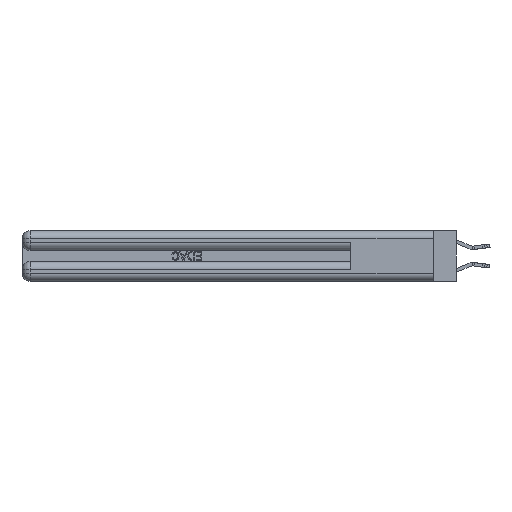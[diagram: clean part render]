
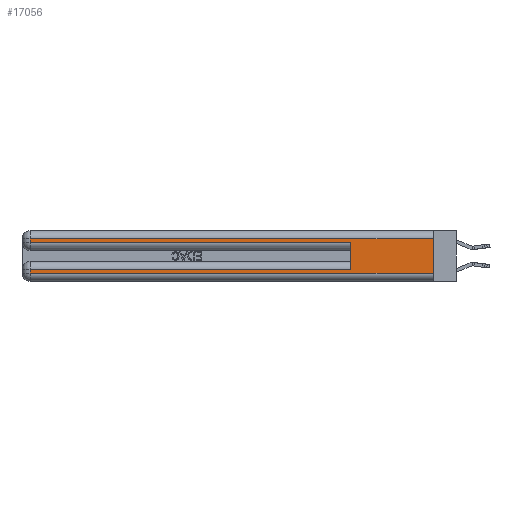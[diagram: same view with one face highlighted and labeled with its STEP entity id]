
A CAD part, left-side view. The second image highlights one B-rep face of the part: STEP entity #17056.
In plain terms, the highlighted planar face has unit normal (-1, 0, 0).
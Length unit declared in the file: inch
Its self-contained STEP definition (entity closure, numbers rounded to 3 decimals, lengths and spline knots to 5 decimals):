
#570 = CARTESIAN_POINT ( 'NONE',  ( 0., 0., 0.31 ) ) ;
#809 = DIRECTION ( 'NONE',  ( 0., -1., 0. ) ) ;
#1093 = LINE ( 'NONE', #29377, #14664 ) ;
#2727 = LINE ( 'NONE', #21797, #16278 ) ;
#3229 = CARTESIAN_POINT ( 'NONE',  ( 0., 0., 0.06 ) ) ;
#5122 = VECTOR ( 'NONE', #32197, 39.37008 ) ;
#5146 = ORIENTED_EDGE ( 'NONE', *, *, #20983, .T. ) ;
#5341 = CARTESIAN_POINT ( 'NONE',  ( 0., 0., 0.37 ) ) ;
#5838 = EDGE_CURVE ( 'NONE', #23781, #7945, #17142, .T. ) ;
#6413 = LINE ( 'NONE', #32430, #27212 ) ;
#6625 = LINE ( 'NONE', #570, #13001 ) ;
#7056 = CARTESIAN_POINT ( 'NONE',  ( 0., 2.94, 0.285 ) ) ;
#7945 = VERTEX_POINT ( 'NONE', #20571 ) ;
#8045 = DIRECTION ( 'NONE',  ( 0., 0., -1. ) ) ;
#8133 = VERTEX_POINT ( 'NONE', #23997 ) ;
#8464 = CARTESIAN_POINT ( 'NONE',  ( 0., 0., 0.285 ) ) ;
#8973 = FACE_OUTER_BOUND ( 'NONE', #31377, .T. ) ;
#9471 = ORIENTED_EDGE ( 'NONE', *, *, #14896, .T. ) ;
#10245 = VERTEX_POINT ( 'NONE', #3229 ) ;
#11460 = CARTESIAN_POINT ( 'NONE',  ( 0., 2.94, 0.085 ) ) ;
#13001 = VECTOR ( 'NONE', #16779, 39.37008 ) ;
#13388 = EDGE_CURVE ( 'NONE', #20049, #7945, #17546, .T. ) ;
#13820 = DIRECTION ( 'NONE',  ( 0., -1., 0. ) ) ;
#14614 = ORIENTED_EDGE ( 'NONE', *, *, #5838, .T. ) ;
#14664 = VECTOR ( 'NONE', #15831, 39.37008 ) ;
#14896 = EDGE_CURVE ( 'NONE', #8133, #23781, #6413, .T. ) ;
#15412 = CARTESIAN_POINT ( 'NONE',  ( 0., 0.6, 0.145 ) ) ;
#15568 = LINE ( 'NONE', #17002, #29161 ) ;
#15618 = EDGE_CURVE ( 'NONE', #28615, #20566, #2727, .T. ) ;
#15831 = DIRECTION ( 'NONE',  ( 0., 0., -1. ) ) ;
#16278 = VECTOR ( 'NONE', #24514, 39.37008 ) ;
#16779 = DIRECTION ( 'NONE',  ( 0., 1., 0. ) ) ;
#17002 = CARTESIAN_POINT ( 'NONE',  ( 0., 0., 0.06 ) ) ;
#17056 = ADVANCED_FACE ( 'NONE', ( #8973 ), #21589, .F. ) ;
#17142 = LINE ( 'NONE', #8464, #24382 ) ;
#17546 = LINE ( 'NONE', #15412, #23959 ) ;
#17814 = LINE ( 'NONE', #29443, #5122 ) ;
#18250 = CARTESIAN_POINT ( 'NONE',  ( 0., 0.6, 0.085 ) ) ;
#18718 = EDGE_CURVE ( 'NONE', #20049, #28615, #17814, .T. ) ;
#19972 = VERTEX_POINT ( 'NONE', #34319 ) ;
#20049 = VERTEX_POINT ( 'NONE', #18250 ) ;
#20566 = VERTEX_POINT ( 'NONE', #31818 ) ;
#20571 = CARTESIAN_POINT ( 'NONE',  ( 0., 0.6, 0.285 ) ) ;
#20983 = EDGE_CURVE ( 'NONE', #20566, #10245, #15568, .T. ) ;
#21589 = PLANE ( 'NONE',  #28433 ) ;
#21797 = CARTESIAN_POINT ( 'NONE',  ( 0., 2.94, 0.37 ) ) ;
#23781 = VERTEX_POINT ( 'NONE', #7056 ) ;
#23959 = VECTOR ( 'NONE', #34409, 39.37008 ) ;
#23997 = CARTESIAN_POINT ( 'NONE',  ( 0., 2.94, 0.31 ) ) ;
#24310 = DIRECTION ( 'NONE',  ( 1., 0., 0. ) ) ;
#24382 = VECTOR ( 'NONE', #13820, 39.37008 ) ;
#24514 = DIRECTION ( 'NONE',  ( 0., 0., -1. ) ) ;
#24574 = ORIENTED_EDGE ( 'NONE', *, *, #25323, .F. ) ;
#24893 = EDGE_CURVE ( 'NONE', #19972, #8133, #6625, .T. ) ;
#25323 = EDGE_CURVE ( 'NONE', #19972, #10245, #1093, .T. ) ;
#27212 = VECTOR ( 'NONE', #35132, 39.37008 ) ;
#27491 = ORIENTED_EDGE ( 'NONE', *, *, #18718, .T. ) ;
#28433 = AXIS2_PLACEMENT_3D ( 'NONE', #5341, #24310, #8045 ) ;
#28615 = VERTEX_POINT ( 'NONE', #11460 ) ;
#28900 = ORIENTED_EDGE ( 'NONE', *, *, #13388, .F. ) ;
#29161 = VECTOR ( 'NONE', #809, 39.37008 ) ;
#29377 = CARTESIAN_POINT ( 'NONE',  ( 0., 0., 0.37 ) ) ;
#29443 = CARTESIAN_POINT ( 'NONE',  ( 0., 0., 0.085 ) ) ;
#31208 = ORIENTED_EDGE ( 'NONE', *, *, #24893, .T. ) ;
#31377 = EDGE_LOOP ( 'NONE', ( #24574, #31208, #9471, #14614, #28900, #27491, #31565, #5146 ) ) ;
#31565 = ORIENTED_EDGE ( 'NONE', *, *, #15618, .T. ) ;
#31818 = CARTESIAN_POINT ( 'NONE',  ( 0., 2.94, 0.06 ) ) ;
#32197 = DIRECTION ( 'NONE',  ( 0., 1., 0. ) ) ;
#32430 = CARTESIAN_POINT ( 'NONE',  ( 0., 2.94, 0.37 ) ) ;
#34319 = CARTESIAN_POINT ( 'NONE',  ( 0., 0., 0.31 ) ) ;
#34409 = DIRECTION ( 'NONE',  ( 0., 0., 1. ) ) ;
#35132 = DIRECTION ( 'NONE',  ( 0., 0., -1. ) ) ;
